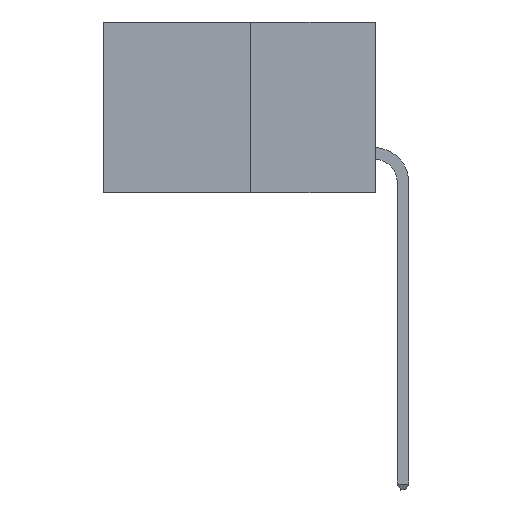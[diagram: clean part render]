
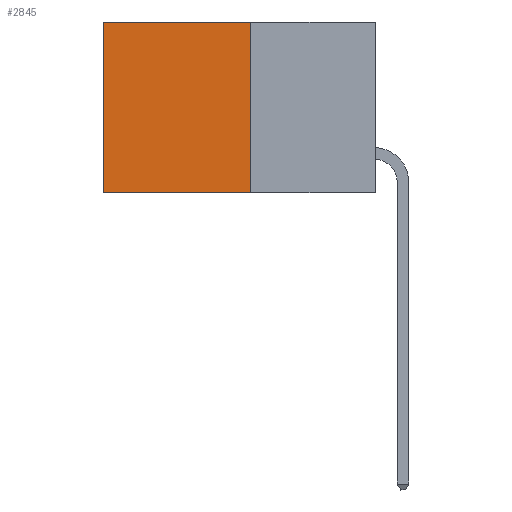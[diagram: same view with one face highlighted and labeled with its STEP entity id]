
A CAD part, left-side view. The second image highlights one B-rep face of the part: STEP entity #2845.
In plain terms, the highlighted planar face has unit normal (-1, 0, 0).
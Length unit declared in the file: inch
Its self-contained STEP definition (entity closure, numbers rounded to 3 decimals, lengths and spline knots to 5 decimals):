
#284 = EDGE_CURVE ( 'NONE', #3758, #2528, #4479, .T. ) ;
#302 = DIRECTION ( 'NONE',  ( 0., 0., -1. ) ) ;
#424 = DIRECTION ( 'NONE',  ( 0., 1., 0. ) ) ;
#925 = DIRECTION ( 'NONE',  ( 0., 1., 0. ) ) ;
#1694 = ORIENTED_EDGE ( 'NONE', *, *, #4951, .F. ) ;
#1942 = DIRECTION ( 'NONE',  ( 1., 0., 0. ) ) ;
#2391 = CARTESIAN_POINT ( 'NONE',  ( 0.277, 0.27, 0. ) ) ;
#2496 = VERTEX_POINT ( 'NONE', #11022 ) ;
#2528 = VERTEX_POINT ( 'NONE', #8787 ) ;
#2707 = PLANE ( 'NONE',  #11719 ) ;
#2845 = ADVANCED_FACE ( 'NONE', ( #3319 ), #2707, .F. ) ;
#3319 = FACE_OUTER_BOUND ( 'NONE', #11361, .T. ) ;
#3323 = VERTEX_POINT ( 'NONE', #6092 ) ;
#3373 = LINE ( 'NONE', #8545, #5600 ) ;
#3758 = VERTEX_POINT ( 'NONE', #9543 ) ;
#4173 = ORIENTED_EDGE ( 'NONE', *, *, #284, .T. ) ;
#4479 = LINE ( 'NONE', #2391, #11431 ) ;
#4503 = CARTESIAN_POINT ( 'NONE',  ( 0.277, 0.27, -0.37 ) ) ;
#4951 = EDGE_CURVE ( 'NONE', #3323, #2496, #5606, .T. ) ;
#5067 = VECTOR ( 'NONE', #424, 39.37008 ) ;
#5222 = LINE ( 'NONE', #4503, #7436 ) ;
#5600 = VECTOR ( 'NONE', #302, 39.37008 ) ;
#5606 = LINE ( 'NONE', #9995, #5067 ) ;
#6092 = CARTESIAN_POINT ( 'NONE',  ( 0.277, 0.27, -0.37 ) ) ;
#7280 = DIRECTION ( 'NONE',  ( 0., 0., -1. ) ) ;
#7436 = VECTOR ( 'NONE', #7280, 39.37008 ) ;
#8512 = ORIENTED_EDGE ( 'NONE', *, *, #8900, .F. ) ;
#8545 = CARTESIAN_POINT ( 'NONE',  ( 0.277, 0.59, -0.37 ) ) ;
#8787 = CARTESIAN_POINT ( 'NONE',  ( 0.277, 0.59, 0. ) ) ;
#8900 = EDGE_CURVE ( 'NONE', #3758, #3323, #5222, .T. ) ;
#9252 = CARTESIAN_POINT ( 'NONE',  ( 0.277, 0.27, -0.37 ) ) ;
#9543 = CARTESIAN_POINT ( 'NONE',  ( 0.277, 0.27, 0. ) ) ;
#9739 = EDGE_CURVE ( 'NONE', #2528, #2496, #3373, .T. ) ;
#9995 = CARTESIAN_POINT ( 'NONE',  ( 0.277, 0.27, -0.37 ) ) ;
#10310 = DIRECTION ( 'NONE',  ( 0., 0., -1. ) ) ;
#11022 = CARTESIAN_POINT ( 'NONE',  ( 0.277, 0.59, -0.37 ) ) ;
#11046 = ORIENTED_EDGE ( 'NONE', *, *, #9739, .T. ) ;
#11361 = EDGE_LOOP ( 'NONE', ( #11046, #1694, #8512, #4173 ) ) ;
#11431 = VECTOR ( 'NONE', #925, 39.37008 ) ;
#11719 = AXIS2_PLACEMENT_3D ( 'NONE', #9252, #1942, #10310 ) ;
